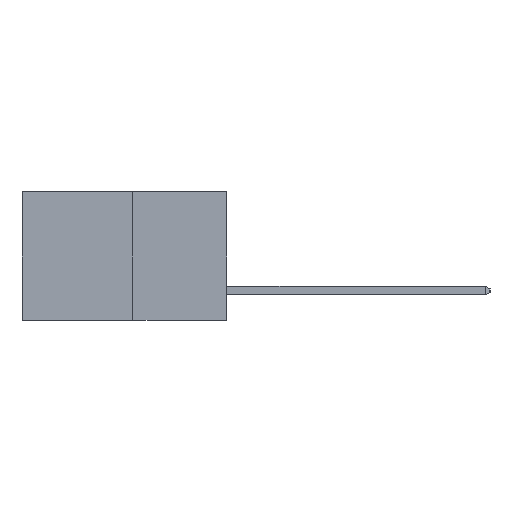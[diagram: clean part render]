
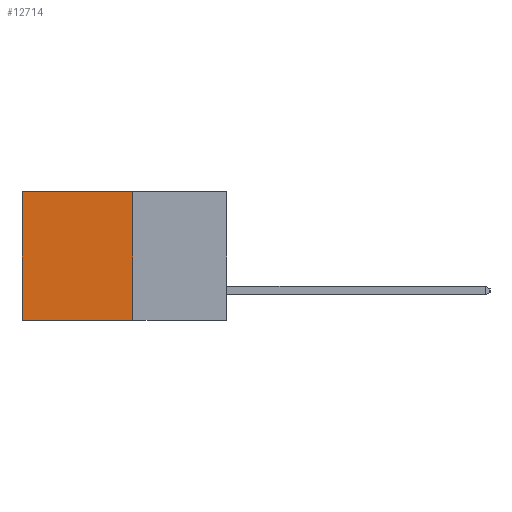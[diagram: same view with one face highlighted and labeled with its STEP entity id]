
A CAD part, left-side view. The second image highlights one B-rep face of the part: STEP entity #12714.
In plain terms, the highlighted planar face has unit normal (-1, 0, 0).
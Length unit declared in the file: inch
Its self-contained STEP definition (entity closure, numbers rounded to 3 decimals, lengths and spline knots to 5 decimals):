
#226 = EDGE_CURVE ( 'NONE', #4642, #3694, #5256, .T. ) ;
#1849 = CARTESIAN_POINT ( 'NONE',  ( 0.277, 0.27, 0. ) ) ;
#2010 = ORIENTED_EDGE ( 'NONE', *, *, #226, .F. ) ;
#2169 = CARTESIAN_POINT ( 'NONE',  ( 0.277, 0.27, -0.37 ) ) ;
#2239 = AXIS2_PLACEMENT_3D ( 'NONE', #4875, #13210, #6969 ) ;
#2365 = VECTOR ( 'NONE', #10584, 39.37008 ) ;
#2382 = ORIENTED_EDGE ( 'NONE', *, *, #9692, .F. ) ;
#2585 = DIRECTION ( 'NONE',  ( 0., 0., -1. ) ) ;
#3215 = CARTESIAN_POINT ( 'NONE',  ( 0.277, 0.27, 0. ) ) ;
#3694 = VERTEX_POINT ( 'NONE', #12322 ) ;
#3725 = CARTESIAN_POINT ( 'NONE',  ( 0.277, 0.59, -0.37 ) ) ;
#4642 = VERTEX_POINT ( 'NONE', #6541 ) ;
#4853 = CARTESIAN_POINT ( 'NONE',  ( 0.277, 0.59, 0. ) ) ;
#4875 = CARTESIAN_POINT ( 'NONE',  ( 0.277, 0.27, -0.37 ) ) ;
#5256 = LINE ( 'NONE', #2169, #2365 ) ;
#5810 = VECTOR ( 'NONE', #9755, 39.37008 ) ;
#6258 = VECTOR ( 'NONE', #2585, 39.37008 ) ;
#6462 = EDGE_LOOP ( 'NONE', ( #12950, #2010, #2382, #11201 ) ) ;
#6541 = CARTESIAN_POINT ( 'NONE',  ( 0.277, 0.27, -0.37 ) ) ;
#6969 = DIRECTION ( 'NONE',  ( 0., 0., -1. ) ) ;
#7397 = VERTEX_POINT ( 'NONE', #4853 ) ;
#7588 = CARTESIAN_POINT ( 'NONE',  ( 0.277, 0.27, -0.37 ) ) ;
#7736 = FACE_OUTER_BOUND ( 'NONE', #6462, .T. ) ;
#8203 = VECTOR ( 'NONE', #9371, 39.37008 ) ;
#8591 = LINE ( 'NONE', #7588, #5810 ) ;
#9371 = DIRECTION ( 'NONE',  ( 0., 1., 0. ) ) ;
#9692 = EDGE_CURVE ( 'NONE', #13639, #4642, #8591, .T. ) ;
#9755 = DIRECTION ( 'NONE',  ( 0., 0., -1. ) ) ;
#10584 = DIRECTION ( 'NONE',  ( 0., 1., 0. ) ) ;
#10890 = LINE ( 'NONE', #3725, #6258 ) ;
#11026 = LINE ( 'NONE', #1849, #8203 ) ;
#11169 = PLANE ( 'NONE',  #2239 ) ;
#11201 = ORIENTED_EDGE ( 'NONE', *, *, #11386, .T. ) ;
#11386 = EDGE_CURVE ( 'NONE', #13639, #7397, #11026, .T. ) ;
#12322 = CARTESIAN_POINT ( 'NONE',  ( 0.277, 0.59, -0.37 ) ) ;
#12659 = EDGE_CURVE ( 'NONE', #7397, #3694, #10890, .T. ) ;
#12714 = ADVANCED_FACE ( 'NONE', ( #7736 ), #11169, .F. ) ;
#12950 = ORIENTED_EDGE ( 'NONE', *, *, #12659, .T. ) ;
#13210 = DIRECTION ( 'NONE',  ( 1., 0., 0. ) ) ;
#13639 = VERTEX_POINT ( 'NONE', #3215 ) ;
